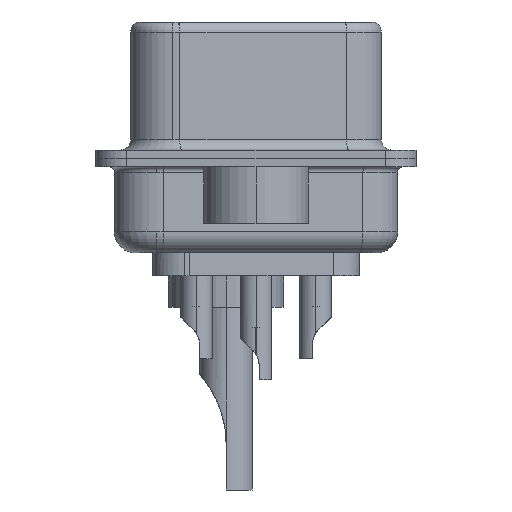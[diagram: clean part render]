
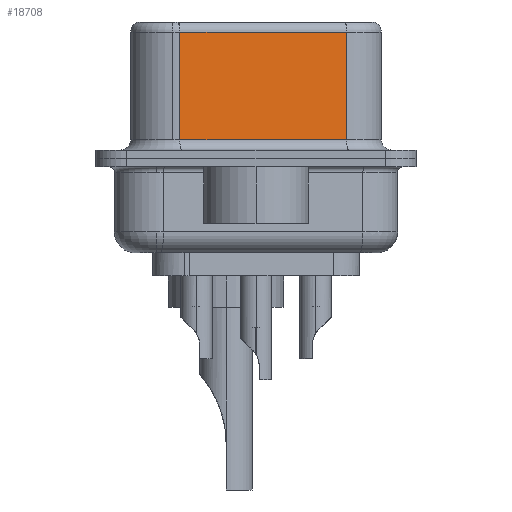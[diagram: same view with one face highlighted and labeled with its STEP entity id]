
A CAD part, left-side view. The second image highlights one B-rep face of the part: STEP entity #18708.
In plain terms, the highlighted planar face has unit normal (-0.985, -0.174, 0).
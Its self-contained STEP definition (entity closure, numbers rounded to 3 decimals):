
#438 = DIRECTION ( 'NONE',  ( 0.174, -0.985, 0. ) ) ;
#441 = FACE_OUTER_BOUND ( 'NONE', #15761, .T. ) ;
#1898 = VECTOR ( 'NONE', #6287, 1000. ) ;
#3051 = AXIS2_PLACEMENT_3D ( 'NONE', #26060, #23858, #10632 ) ;
#3282 = VERTEX_POINT ( 'NONE', #22662 ) ;
#6287 = DIRECTION ( 'NONE',  ( 0., 0., -1. ) ) ;
#6777 = VERTEX_POINT ( 'NONE', #28717 ) ;
#7716 = LINE ( 'NONE', #23835, #1898 ) ;
#8078 = CARTESIAN_POINT ( 'NONE',  ( 5.132, -4.322, 0.9 ) ) ;
#8425 = PLANE ( 'NONE',  #3051 ) ;
#10632 = DIRECTION ( 'NONE',  ( -0.174, 0.985, 0. ) ) ;
#11142 = LINE ( 'NONE', #23444, #22168 ) ;
#11152 = ORIENTED_EDGE ( 'NONE', *, *, #16523, .T. ) ;
#12627 = VERTEX_POINT ( 'NONE', #8078 ) ;
#14728 = EDGE_CURVE ( 'NONE', #19435, #12627, #25524, .T. ) ;
#15011 = CARTESIAN_POINT ( 'NONE',  ( 3.73, 3.628, 6.52 ) ) ;
#15761 = EDGE_LOOP ( 'NONE', ( #20114, #21914, #11152, #17839 ) ) ;
#16523 = EDGE_CURVE ( 'NONE', #3282, #19435, #18730, .T. ) ;
#17839 = ORIENTED_EDGE ( 'NONE', *, *, #14728, .T. ) ;
#18022 = VECTOR ( 'NONE', #28514, 1000. ) ;
#18708 = ADVANCED_FACE ( 'NONE', ( #441 ), #8425, .F. ) ;
#18730 = LINE ( 'NONE', #15011, #18022 ) ;
#19435 = VERTEX_POINT ( 'NONE', #19772 ) ;
#19495 = VECTOR ( 'NONE', #438, 1000. ) ;
#19772 = CARTESIAN_POINT ( 'NONE',  ( 3.73, 3.628, 0.9 ) ) ;
#20114 = ORIENTED_EDGE ( 'NONE', *, *, #22756, .F. ) ;
#21165 = DIRECTION ( 'NONE',  ( -0.174, 0.985, 0. ) ) ;
#21914 = ORIENTED_EDGE ( 'NONE', *, *, #22628, .T. ) ;
#22168 = VECTOR ( 'NONE', #21165, 1000. ) ;
#22628 = EDGE_CURVE ( 'NONE', #6777, #3282, #11142, .T. ) ;
#22662 = CARTESIAN_POINT ( 'NONE',  ( 3.73, 3.628, 6.02 ) ) ;
#22756 = EDGE_CURVE ( 'NONE', #6777, #12627, #7716, .T. ) ;
#23444 = CARTESIAN_POINT ( 'NONE',  ( 5.132, -4.322, 6.02 ) ) ;
#23835 = CARTESIAN_POINT ( 'NONE',  ( 5.132, -4.322, 6.52 ) ) ;
#23858 = DIRECTION ( 'NONE',  ( 0.985, 0.174, 0. ) ) ;
#24611 = CARTESIAN_POINT ( 'NONE',  ( 5.132, -4.322, 0.9 ) ) ;
#25524 = LINE ( 'NONE', #24611, #19495 ) ;
#26060 = CARTESIAN_POINT ( 'NONE',  ( 5.132, -4.322, 6.52 ) ) ;
#28514 = DIRECTION ( 'NONE',  ( 0., 0., -1. ) ) ;
#28717 = CARTESIAN_POINT ( 'NONE',  ( 5.132, -4.322, 6.02 ) ) ;
